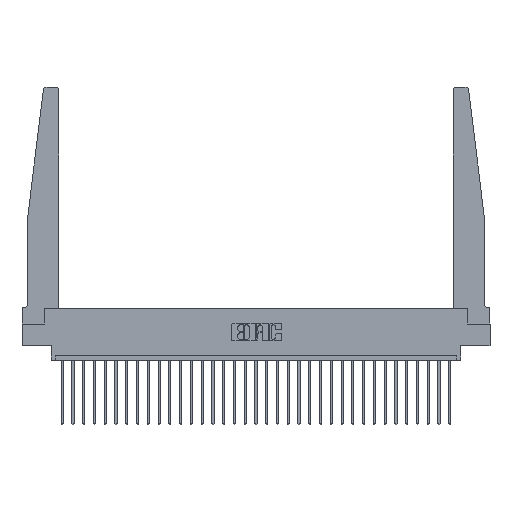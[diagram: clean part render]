
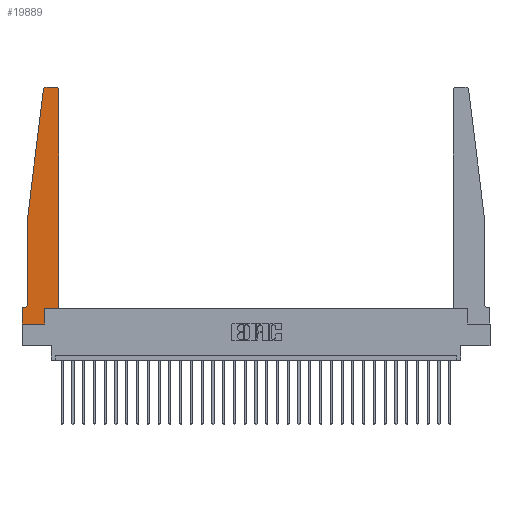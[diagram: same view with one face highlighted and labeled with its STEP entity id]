
A CAD part, top view. The second image highlights one B-rep face of the part: STEP entity #19889.
In plain terms, the highlighted planar face has unit normal (0, 0, 1).
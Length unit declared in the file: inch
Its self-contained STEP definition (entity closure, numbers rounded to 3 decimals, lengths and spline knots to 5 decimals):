
#54 = VERTEX_POINT ( 'NONE', #9262 ) ;
#82 = DIRECTION ( 'NONE',  ( 0., 0., 1. ) ) ;
#633 = CIRCLE ( 'NONE', #11470, 0.03 ) ;
#781 = LINE ( 'NONE', #2954, #22437 ) ;
#1142 = CARTESIAN_POINT ( 'NONE',  ( 0., 0.1875, 0.37 ) ) ;
#1172 = AXIS2_PLACEMENT_3D ( 'NONE', #13088, #26127, #8660 ) ;
#1301 = CARTESIAN_POINT ( 'NONE',  ( 0.425, 2.72, 0.37 ) ) ;
#1420 = VECTOR ( 'NONE', #5750, 39.37008 ) ;
#1510 = VERTEX_POINT ( 'NONE', #10412 ) ;
#2615 = CARTESIAN_POINT ( 'NONE',  ( 0., 0., 0.37 ) ) ;
#2622 = FACE_OUTER_BOUND ( 'NONE', #28807, .T. ) ;
#2954 = CARTESIAN_POINT ( 'NONE',  ( 0.065, 0.1875, 0.37 ) ) ;
#2979 = CARTESIAN_POINT ( 'NONE',  ( 0.425, 0.18, 0.37 ) ) ;
#3122 = VECTOR ( 'NONE', #8386, 39.37008 ) ;
#3401 = CARTESIAN_POINT ( 'NONE',  ( 0.065, 1.25, 0.37 ) ) ;
#3432 = EDGE_CURVE ( 'NONE', #5364, #3561, #19477, .T. ) ;
#3524 = LINE ( 'NONE', #19246, #1420 ) ;
#3561 = VERTEX_POINT ( 'NONE', #23276 ) ;
#3586 = DIRECTION ( 'NONE',  ( 1., 0., 0. ) ) ;
#4925 = EDGE_CURVE ( 'NONE', #54, #14072, #23586, .T. ) ;
#5035 = LINE ( 'NONE', #2615, #22726 ) ;
#5093 = AXIS2_PLACEMENT_3D ( 'NONE', #11948, #21015, #11645 ) ;
#5312 = VERTEX_POINT ( 'NONE', #6033 ) ;
#5364 = VERTEX_POINT ( 'NONE', #1301 ) ;
#5377 = EDGE_CURVE ( 'NONE', #1510, #19115, #3524, .T. ) ;
#5570 = VECTOR ( 'NONE', #28061, 39.37008 ) ;
#5750 = DIRECTION ( 'NONE',  ( 1., 0., 0. ) ) ;
#5888 = CARTESIAN_POINT ( 'NONE',  ( 0.015, 0.1875, 0.37 ) ) ;
#6033 = CARTESIAN_POINT ( 'NONE',  ( 0.24675, 2.72367, 0.37 ) ) ;
#6100 = ORIENTED_EDGE ( 'NONE', *, *, #21461, .T. ) ;
#6162 = LINE ( 'NONE', #17335, #3122 ) ;
#6671 = ORIENTED_EDGE ( 'NONE', *, *, #28825, .T. ) ;
#6991 = ORIENTED_EDGE ( 'NONE', *, *, #26893, .T. ) ;
#7163 = DIRECTION ( 'NONE',  ( 1., 0., 0. ) ) ;
#8386 = DIRECTION ( 'NONE',  ( 0., 1., 0. ) ) ;
#8620 = EDGE_CURVE ( 'NONE', #16731, #17765, #23549, .T. ) ;
#8660 = DIRECTION ( 'NONE',  ( 1., 0., 0. ) ) ;
#9032 = DIRECTION ( 'NONE',  ( 0., -1., 0. ) ) ;
#9262 = CARTESIAN_POINT ( 'NONE',  ( 0.2605, 0.18, 0.37 ) ) ;
#9905 = ORIENTED_EDGE ( 'NONE', *, *, #11892, .T. ) ;
#10187 = VECTOR ( 'NONE', #3586, 39.37008 ) ;
#10412 = CARTESIAN_POINT ( 'NONE',  ( 0., 0., 0.37 ) ) ;
#10853 = ORIENTED_EDGE ( 'NONE', *, *, #28153, .T. ) ;
#10921 = DIRECTION ( 'NONE',  ( -0.122, -0.992, 0. ) ) ;
#11470 = AXIS2_PLACEMENT_3D ( 'NONE', #20487, #82, #25052 ) ;
#11645 = DIRECTION ( 'NONE',  ( -1., 0., 0. ) ) ;
#11729 = ORIENTED_EDGE ( 'NONE', *, *, #23217, .T. ) ;
#11892 = EDGE_CURVE ( 'NONE', #19115, #54, #16583, .T. ) ;
#11948 = CARTESIAN_POINT ( 'NONE',  ( 0.015, 0.2375, 0.37 ) ) ;
#13088 = CARTESIAN_POINT ( 'NONE',  ( 0.395, 2.72, 0.37 ) ) ;
#13623 = ORIENTED_EDGE ( 'NONE', *, *, #5377, .T. ) ;
#13884 = CARTESIAN_POINT ( 'NONE',  ( 0., 0.1875, 0.37 ) ) ;
#14072 = VERTEX_POINT ( 'NONE', #26972 ) ;
#14741 = AXIS2_PLACEMENT_3D ( 'NONE', #13884, #27199, #7163 ) ;
#15368 = CARTESIAN_POINT ( 'NONE',  ( 0.065, 1.25, 0.37 ) ) ;
#15825 = VERTEX_POINT ( 'NONE', #5888 ) ;
#15929 = CIRCLE ( 'NONE', #5093, 0.05 ) ;
#16356 = ORIENTED_EDGE ( 'NONE', *, *, #4925, .T. ) ;
#16583 = LINE ( 'NONE', #23730, #26228 ) ;
#16731 = VERTEX_POINT ( 'NONE', #27095 ) ;
#16871 = CARTESIAN_POINT ( 'NONE',  ( 0.27653, 2.75, 0.37 ) ) ;
#16991 = DIRECTION ( 'NONE',  ( -1., 0., 0. ) ) ;
#17335 = CARTESIAN_POINT ( 'NONE',  ( 0.425, 0.18, 0.37 ) ) ;
#17765 = VERTEX_POINT ( 'NONE', #18918 ) ;
#18273 = PLANE ( 'NONE',  #14741 ) ;
#18918 = CARTESIAN_POINT ( 'NONE',  ( 0.065, 0.2375, 0.37 ) ) ;
#19030 = ORIENTED_EDGE ( 'NONE', *, *, #22005, .T. ) ;
#19115 = VERTEX_POINT ( 'NONE', #23935 ) ;
#19246 = CARTESIAN_POINT ( 'NONE',  ( 0., 0., 0.37 ) ) ;
#19257 = CARTESIAN_POINT ( 'NONE',  ( 0.25, 2.75, 0.37 ) ) ;
#19477 = CIRCLE ( 'NONE', #1172, 0.03 ) ;
#19686 = ORIENTED_EDGE ( 'NONE', *, *, #28894, .T. ) ;
#19889 = ADVANCED_FACE ( 'NONE', ( #2622 ), #18273, .T. ) ;
#20487 = CARTESIAN_POINT ( 'NONE',  ( 0.27653, 2.72, 0.37 ) ) ;
#21015 = DIRECTION ( 'NONE',  ( 0., 0., -1. ) ) ;
#21461 = EDGE_CURVE ( 'NONE', #3561, #25702, #23976, .T. ) ;
#22005 = EDGE_CURVE ( 'NONE', #22886, #1510, #5035, .T. ) ;
#22437 = VECTOR ( 'NONE', #16991, 39.37008 ) ;
#22726 = VECTOR ( 'NONE', #9032, 39.37008 ) ;
#22778 = ORIENTED_EDGE ( 'NONE', *, *, #8620, .T. ) ;
#22886 = VERTEX_POINT ( 'NONE', #1142 ) ;
#23217 = EDGE_CURVE ( 'NONE', #25702, #5312, #633, .T. ) ;
#23276 = CARTESIAN_POINT ( 'NONE',  ( 0.395, 2.75, 0.37 ) ) ;
#23549 = LINE ( 'NONE', #3401, #5570 ) ;
#23586 = LINE ( 'NONE', #2979, #10187 ) ;
#23730 = CARTESIAN_POINT ( 'NONE',  ( 0.2605, 0.18, 0.37 ) ) ;
#23935 = CARTESIAN_POINT ( 'NONE',  ( 0.2605, 0., 0.37 ) ) ;
#23976 = LINE ( 'NONE', #19257, #24126 ) ;
#24126 = VECTOR ( 'NONE', #26326, 39.37008 ) ;
#25052 = DIRECTION ( 'NONE',  ( 1., 0., 0. ) ) ;
#25234 = ORIENTED_EDGE ( 'NONE', *, *, #3432, .T. ) ;
#25524 = DIRECTION ( 'NONE',  ( 0., 1., 0. ) ) ;
#25702 = VERTEX_POINT ( 'NONE', #16871 ) ;
#26127 = DIRECTION ( 'NONE',  ( 0., 0., 1. ) ) ;
#26228 = VECTOR ( 'NONE', #25524, 39.37008 ) ;
#26326 = DIRECTION ( 'NONE',  ( -1., 0., 0. ) ) ;
#26654 = VECTOR ( 'NONE', #10921, 39.37008 ) ;
#26760 = LINE ( 'NONE', #15368, #26654 ) ;
#26893 = EDGE_CURVE ( 'NONE', #15825, #22886, #781, .T. ) ;
#26972 = CARTESIAN_POINT ( 'NONE',  ( 0.425, 0.18, 0.37 ) ) ;
#27095 = CARTESIAN_POINT ( 'NONE',  ( 0.065, 1.25, 0.37 ) ) ;
#27199 = DIRECTION ( 'NONE',  ( 0., 0., 1. ) ) ;
#28061 = DIRECTION ( 'NONE',  ( 0., -1., 0. ) ) ;
#28153 = EDGE_CURVE ( 'NONE', #14072, #5364, #6162, .T. ) ;
#28807 = EDGE_LOOP ( 'NONE', ( #6100, #11729, #6671, #22778, #19686, #6991, #19030, #13623, #9905, #16356, #10853, #25234 ) ) ;
#28825 = EDGE_CURVE ( 'NONE', #5312, #16731, #26760, .T. ) ;
#28894 = EDGE_CURVE ( 'NONE', #17765, #15825, #15929, .T. ) ;
